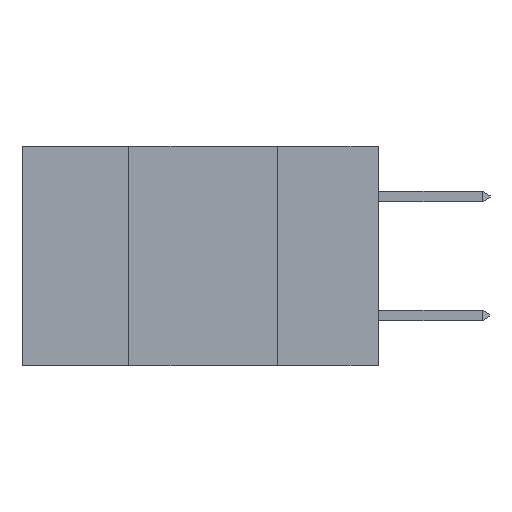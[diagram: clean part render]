
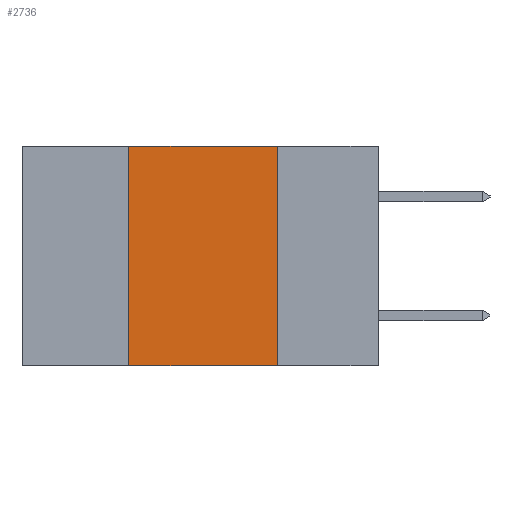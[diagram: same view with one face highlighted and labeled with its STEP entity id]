
A CAD part, left-side view. The second image highlights one B-rep face of the part: STEP entity #2736.
In plain terms, the highlighted planar face has unit normal (-1, 0, 0).
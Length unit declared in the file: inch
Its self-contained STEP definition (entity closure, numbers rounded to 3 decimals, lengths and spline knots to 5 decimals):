
#52 = CARTESIAN_POINT ( 'NONE',  ( 0., 0.6, 0. ) ) ;
#480 = ORIENTED_EDGE ( 'NONE', *, *, #4141, .T. ) ;
#685 = FACE_OUTER_BOUND ( 'NONE', #3478, .T. ) ;
#696 = VERTEX_POINT ( 'NONE', #7048 ) ;
#777 = DIRECTION ( 'NONE',  ( 1., 0., 0. ) ) ;
#2104 = VECTOR ( 'NONE', #10870, 39.37008 ) ;
#2363 = VECTOR ( 'NONE', #11511, 39.37008 ) ;
#2661 = LINE ( 'NONE', #8350, #3437 ) ;
#2736 = ADVANCED_FACE ( 'NONE', ( #685 ), #9438, .F. ) ;
#2832 = VECTOR ( 'NONE', #7817, 39.37008 ) ;
#3437 = VECTOR ( 'NONE', #7462, 39.37008 ) ;
#3478 = EDGE_LOOP ( 'NONE', ( #8727, #8453, #12260, #480 ) ) ;
#3577 = CARTESIAN_POINT ( 'NONE',  ( 0., 0.17, -0.37 ) ) ;
#4141 = EDGE_CURVE ( 'NONE', #9502, #7423, #2661, .T. ) ;
#4960 = LINE ( 'NONE', #52, #2832 ) ;
#5729 = AXIS2_PLACEMENT_3D ( 'NONE', #11349, #777, #8417 ) ;
#6241 = EDGE_CURVE ( 'NONE', #696, #6368, #4960, .T. ) ;
#6368 = VERTEX_POINT ( 'NONE', #11708 ) ;
#7048 = CARTESIAN_POINT ( 'NONE',  ( 0., 0.42, 0. ) ) ;
#7208 = EDGE_CURVE ( 'NONE', #6368, #7423, #7654, .T. ) ;
#7423 = VERTEX_POINT ( 'NONE', #3577 ) ;
#7462 = DIRECTION ( 'NONE',  ( 0., -1., 0. ) ) ;
#7654 = LINE ( 'NONE', #11450, #2363 ) ;
#7817 = DIRECTION ( 'NONE',  ( 0., -1., 0. ) ) ;
#8012 = LINE ( 'NONE', #8888, #2104 ) ;
#8350 = CARTESIAN_POINT ( 'NONE',  ( 0., 0.6, -0.37 ) ) ;
#8417 = DIRECTION ( 'NONE',  ( 0., 0., -1. ) ) ;
#8453 = ORIENTED_EDGE ( 'NONE', *, *, #6241, .F. ) ;
#8727 = ORIENTED_EDGE ( 'NONE', *, *, #7208, .F. ) ;
#8888 = CARTESIAN_POINT ( 'NONE',  ( 0., 0.42, -0.37 ) ) ;
#9438 = PLANE ( 'NONE',  #5729 ) ;
#9502 = VERTEX_POINT ( 'NONE', #11702 ) ;
#10560 = EDGE_CURVE ( 'NONE', #9502, #696, #8012, .T. ) ;
#10870 = DIRECTION ( 'NONE',  ( 0., 0., 1. ) ) ;
#11349 = CARTESIAN_POINT ( 'NONE',  ( 0., 0.6, 0. ) ) ;
#11450 = CARTESIAN_POINT ( 'NONE',  ( 0., 0.17, -0.37 ) ) ;
#11511 = DIRECTION ( 'NONE',  ( 0., 0., -1. ) ) ;
#11702 = CARTESIAN_POINT ( 'NONE',  ( 0., 0.42, -0.37 ) ) ;
#11708 = CARTESIAN_POINT ( 'NONE',  ( 0., 0.17, 0. ) ) ;
#12260 = ORIENTED_EDGE ( 'NONE', *, *, #10560, .F. ) ;
